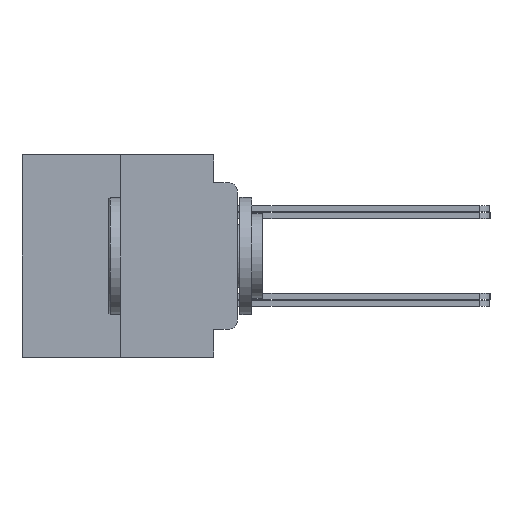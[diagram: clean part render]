
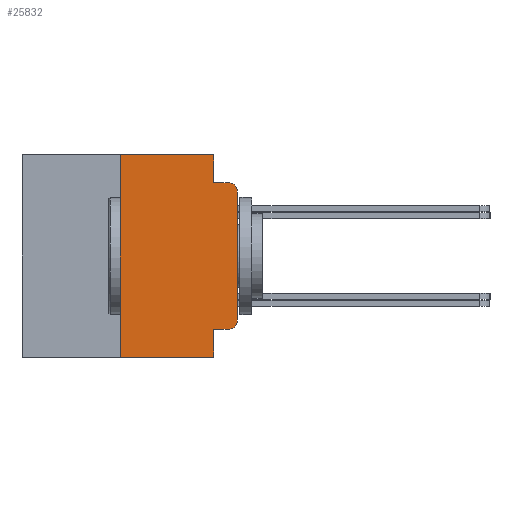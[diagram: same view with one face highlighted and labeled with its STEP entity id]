
A CAD part, left-side view. The second image highlights one B-rep face of the part: STEP entity #25832.
In plain terms, the highlighted planar face has unit normal (-1, 0, 0).
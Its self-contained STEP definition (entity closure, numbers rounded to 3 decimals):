
#92 = EDGE_CURVE ( 'NONE', #22735, #12809, #15053, .T. ) ;
#578 = AXIS2_PLACEMENT_3D ( 'NONE', #27060, #13360, #1981 ) ;
#986 = VECTOR ( 'NONE', #2826, 1000. ) ;
#1981 = DIRECTION ( 'NONE',  ( 0., 0., -1. ) ) ;
#2826 = DIRECTION ( 'NONE',  ( 0., -1., 0. ) ) ;
#3185 = CARTESIAN_POINT ( 'NONE',  ( -75.603, 0.508, -3.975 ) ) ;
#3914 = CARTESIAN_POINT ( 'NONE',  ( -75.603, 6.35, -5.486 ) ) ;
#5010 = FACE_OUTER_BOUND ( 'NONE', #16758, .T. ) ;
#5015 = EDGE_CURVE ( 'NONE', #29354, #23358, #16662, .T. ) ;
#5410 = VECTOR ( 'NONE', #27323, 1000. ) ;
#5536 = CARTESIAN_POINT ( 'NONE',  ( -75.603, 0., 3.467 ) ) ;
#5628 = EDGE_CURVE ( 'NONE', #9155, #12809, #13758, .T. ) ;
#6050 = LINE ( 'NONE', #23496, #986 ) ;
#6486 = DIRECTION ( 'NONE',  ( 0., 0., -1. ) ) ;
#7334 = CARTESIAN_POINT ( 'NONE',  ( -75.603, 1.295, 3.975 ) ) ;
#7993 = DIRECTION ( 'NONE',  ( 0., 0., -1. ) ) ;
#8096 = CARTESIAN_POINT ( 'NONE',  ( -75.603, 1.295, 0. ) ) ;
#8193 = EDGE_CURVE ( 'NONE', #23358, #12409, #24486, .T. ) ;
#8512 = DIRECTION ( 'NONE',  ( 0., 0., 1. ) ) ;
#8534 = CARTESIAN_POINT ( 'NONE',  ( -75.603, 1.295, -3.975 ) ) ;
#8927 = VERTEX_POINT ( 'NONE', #26984 ) ;
#9066 = VERTEX_POINT ( 'NONE', #25512 ) ;
#9155 = VERTEX_POINT ( 'NONE', #5536 ) ;
#9842 = ORIENTED_EDGE ( 'NONE', *, *, #19275, .F. ) ;
#10313 = AXIS2_PLACEMENT_3D ( 'NONE', #10701, #26804, #21995 ) ;
#10413 = VECTOR ( 'NONE', #8512, 1000. ) ;
#10701 = CARTESIAN_POINT ( 'NONE',  ( -75.603, 0.508, -3.467 ) ) ;
#11051 = PLANE ( 'NONE',  #578 ) ;
#11432 = DIRECTION ( 'NONE',  ( -1., 0., 0. ) ) ;
#11468 = ORIENTED_EDGE ( 'NONE', *, *, #8193, .T. ) ;
#12409 = VERTEX_POINT ( 'NONE', #23036 ) ;
#12809 = VERTEX_POINT ( 'NONE', #19708 ) ;
#13360 = DIRECTION ( 'NONE',  ( 1., 0., 0. ) ) ;
#13431 = CARTESIAN_POINT ( 'NONE',  ( -75.603, 0., 5.486 ) ) ;
#13558 = CARTESIAN_POINT ( 'NONE',  ( -75.603, 6.35, 5.486 ) ) ;
#13758 = CIRCLE ( 'NONE', #15058, 0.508 ) ;
#13932 = CARTESIAN_POINT ( 'NONE',  ( -75.603, 1.295, 3.975 ) ) ;
#13974 = EDGE_CURVE ( 'NONE', #17177, #25763, #16509, .T. ) ;
#14433 = DIRECTION ( 'NONE',  ( 0., -1., 0. ) ) ;
#14752 = CARTESIAN_POINT ( 'NONE',  ( -75.603, 1.295, 0. ) ) ;
#15053 = LINE ( 'NONE', #13932, #25750 ) ;
#15058 = AXIS2_PLACEMENT_3D ( 'NONE', #18235, #11432, #6486 ) ;
#15180 = DIRECTION ( 'NONE',  ( 0., -1., 0. ) ) ;
#15236 = DIRECTION ( 'NONE',  ( 0., 0., -1. ) ) ;
#15275 = CARTESIAN_POINT ( 'NONE',  ( -75.603, 6.35, -5.486 ) ) ;
#15977 = CARTESIAN_POINT ( 'NONE',  ( -75.603, 1.295, -3.975 ) ) ;
#16509 = LINE ( 'NONE', #15275, #10413 ) ;
#16662 = LINE ( 'NONE', #15977, #26318 ) ;
#16758 = EDGE_LOOP ( 'NONE', ( #24626, #11468, #22666, #29207, #18959, #9842, #20847, #23487, #24192, #20157 ) ) ;
#17177 = VERTEX_POINT ( 'NONE', #3914 ) ;
#17201 = LINE ( 'NONE', #14752, #27220 ) ;
#18235 = CARTESIAN_POINT ( 'NONE',  ( -75.603, 0.508, 3.467 ) ) ;
#18775 = EDGE_CURVE ( 'NONE', #17177, #9066, #28320, .T. ) ;
#18959 = ORIENTED_EDGE ( 'NONE', *, *, #92, .F. ) ;
#18971 = LINE ( 'NONE', #13431, #5410 ) ;
#19015 = VECTOR ( 'NONE', #15180, 1000. ) ;
#19275 = EDGE_CURVE ( 'NONE', #8927, #22735, #17201, .T. ) ;
#19708 = CARTESIAN_POINT ( 'NONE',  ( -75.603, 0.508, 3.975 ) ) ;
#20157 = ORIENTED_EDGE ( 'NONE', *, *, #26177, .F. ) ;
#20847 = ORIENTED_EDGE ( 'NONE', *, *, #26624, .F. ) ;
#21995 = DIRECTION ( 'NONE',  ( 0., 0., -1. ) ) ;
#22666 = ORIENTED_EDGE ( 'NONE', *, *, #28932, .T. ) ;
#22735 = VERTEX_POINT ( 'NONE', #7334 ) ;
#22757 = DIRECTION ( 'NONE',  ( 0., -1., 0. ) ) ;
#23036 = CARTESIAN_POINT ( 'NONE',  ( -75.603, 0., -3.467 ) ) ;
#23358 = VERTEX_POINT ( 'NONE', #3185 ) ;
#23487 = ORIENTED_EDGE ( 'NONE', *, *, #13974, .F. ) ;
#23496 = CARTESIAN_POINT ( 'NONE',  ( -75.603, 11.684, 5.486 ) ) ;
#24185 = CARTESIAN_POINT ( 'NONE',  ( -75.603, 11.684, -5.486 ) ) ;
#24192 = ORIENTED_EDGE ( 'NONE', *, *, #18775, .T. ) ;
#24486 = CIRCLE ( 'NONE', #10313, 0.508 ) ;
#24626 = ORIENTED_EDGE ( 'NONE', *, *, #5015, .T. ) ;
#25324 = VECTOR ( 'NONE', #15236, 1000. ) ;
#25512 = CARTESIAN_POINT ( 'NONE',  ( -75.603, 1.295, -5.486 ) ) ;
#25750 = VECTOR ( 'NONE', #14433, 1000. ) ;
#25763 = VERTEX_POINT ( 'NONE', #13558 ) ;
#25832 = ADVANCED_FACE ( 'NONE', ( #5010 ), #11051, .F. ) ;
#26177 = EDGE_CURVE ( 'NONE', #29354, #9066, #26407, .T. ) ;
#26318 = VECTOR ( 'NONE', #22757, 1000. ) ;
#26407 = LINE ( 'NONE', #8096, #25324 ) ;
#26624 = EDGE_CURVE ( 'NONE', #25763, #8927, #6050, .T. ) ;
#26804 = DIRECTION ( 'NONE',  ( -1., 0., 0. ) ) ;
#26984 = CARTESIAN_POINT ( 'NONE',  ( -75.603, 1.295, 5.486 ) ) ;
#27060 = CARTESIAN_POINT ( 'NONE',  ( -75.603, 11.684, 5.486 ) ) ;
#27220 = VECTOR ( 'NONE', #7993, 1000. ) ;
#27323 = DIRECTION ( 'NONE',  ( 0., 0., 1. ) ) ;
#28320 = LINE ( 'NONE', #24185, #19015 ) ;
#28932 = EDGE_CURVE ( 'NONE', #12409, #9155, #18971, .T. ) ;
#29207 = ORIENTED_EDGE ( 'NONE', *, *, #5628, .T. ) ;
#29354 = VERTEX_POINT ( 'NONE', #8534 ) ;
